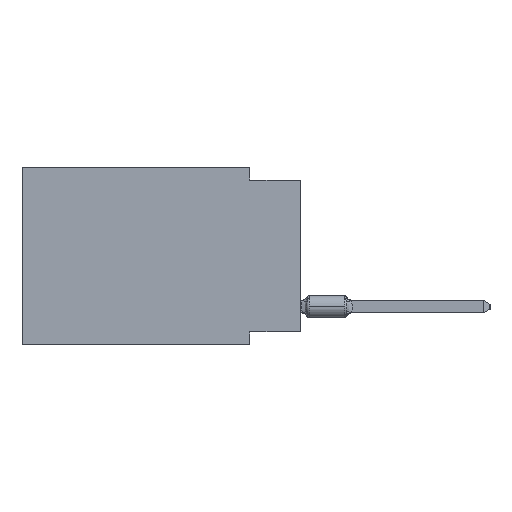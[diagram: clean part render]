
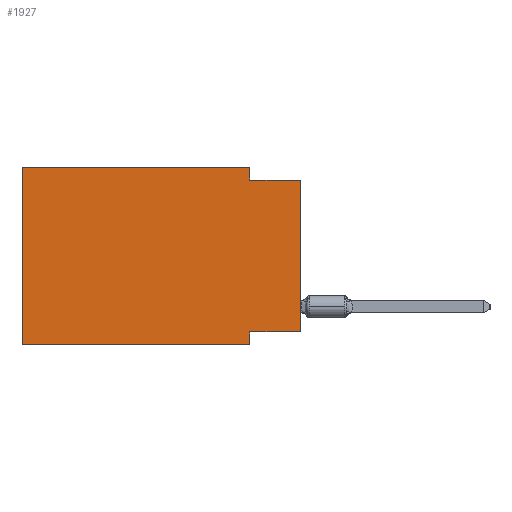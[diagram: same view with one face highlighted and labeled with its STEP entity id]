
A CAD part, left-side view. The second image highlights one B-rep face of the part: STEP entity #1927.
In plain terms, the highlighted planar face has unit normal (-1, 0, 0).
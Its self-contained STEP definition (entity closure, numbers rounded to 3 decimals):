
#405 = CARTESIAN_POINT ( 'NONE',  ( 0., 13.97, 0. ) ) ;
#602 = VECTOR ( 'NONE', #10514, 1000. ) ;
#1927 = ADVANCED_FACE ( 'NONE', ( #8157 ), #25574, .F. ) ;
#2045 = AXIS2_PLACEMENT_3D ( 'NONE', #12859, #8433, #4004 ) ;
#3467 = EDGE_CURVE ( 'NONE', #17275, #5805, #4406, .T. ) ;
#3795 = ORIENTED_EDGE ( 'NONE', *, *, #14991, .F. ) ;
#3963 = DIRECTION ( 'NONE',  ( 0., -1., 0. ) ) ;
#4004 = DIRECTION ( 'NONE',  ( 0., 0., -1. ) ) ;
#4112 = ORIENTED_EDGE ( 'NONE', *, *, #22941, .F. ) ;
#4251 = EDGE_CURVE ( 'NONE', #5805, #24620, #11693, .T. ) ;
#4406 = LINE ( 'NONE', #10503, #20689 ) ;
#4464 = ORIENTED_EDGE ( 'NONE', *, *, #23027, .F. ) ;
#4549 = LINE ( 'NONE', #8986, #602 ) ;
#4824 = CARTESIAN_POINT ( 'NONE',  ( 0., 2.54, -8.89 ) ) ;
#5795 = LINE ( 'NONE', #10486, #11749 ) ;
#5805 = VERTEX_POINT ( 'NONE', #18101 ) ;
#6042 = LINE ( 'NONE', #22933, #11833 ) ;
#6644 = VECTOR ( 'NONE', #8421, 1000. ) ;
#7253 = VECTOR ( 'NONE', #12324, 1000. ) ;
#7646 = ORIENTED_EDGE ( 'NONE', *, *, #23151, .T. ) ;
#7904 = CARTESIAN_POINT ( 'NONE',  ( 0., 2.54, 0. ) ) ;
#8157 = FACE_OUTER_BOUND ( 'NONE', #25905, .T. ) ;
#8173 = LINE ( 'NONE', #7904, #7253 ) ;
#8421 = DIRECTION ( 'NONE',  ( 0., 0., 1. ) ) ;
#8433 = DIRECTION ( 'NONE',  ( 1., 0., 0. ) ) ;
#8986 = CARTESIAN_POINT ( 'NONE',  ( 0., 13.97, -8.89 ) ) ;
#10387 = ORIENTED_EDGE ( 'NONE', *, *, #24903, .T. ) ;
#10486 = CARTESIAN_POINT ( 'NONE',  ( 0., 0., 0. ) ) ;
#10503 = CARTESIAN_POINT ( 'NONE',  ( 0., 0., -8.255 ) ) ;
#10514 = DIRECTION ( 'NONE',  ( 0., -1., 0. ) ) ;
#11693 = LINE ( 'NONE', #15861, #21605 ) ;
#11749 = VECTOR ( 'NONE', #27346, 1000. ) ;
#11811 = ORIENTED_EDGE ( 'NONE', *, *, #4251, .F. ) ;
#11833 = VECTOR ( 'NONE', #3963, 1000. ) ;
#12324 = DIRECTION ( 'NONE',  ( 0., 0., -1. ) ) ;
#12859 = CARTESIAN_POINT ( 'NONE',  ( 0., 13.97, 0. ) ) ;
#12860 = DIRECTION ( 'NONE',  ( 0., 1., 0. ) ) ;
#14485 = CARTESIAN_POINT ( 'NONE',  ( 0., 2.54, -0.635 ) ) ;
#14671 = DIRECTION ( 'NONE',  ( 0., -1., 0. ) ) ;
#14783 = CARTESIAN_POINT ( 'NONE',  ( 0., 13.97, 0. ) ) ;
#14882 = VERTEX_POINT ( 'NONE', #14485 ) ;
#14991 = EDGE_CURVE ( 'NONE', #18155, #26142, #6042, .T. ) ;
#15861 = CARTESIAN_POINT ( 'NONE',  ( 0., 2.54, -8.89 ) ) ;
#16472 = LINE ( 'NONE', #22581, #19612 ) ;
#16500 = CARTESIAN_POINT ( 'NONE',  ( 0., 0., -0.635 ) ) ;
#17275 = VERTEX_POINT ( 'NONE', #23997 ) ;
#18101 = CARTESIAN_POINT ( 'NONE',  ( 0., 2.54, -8.255 ) ) ;
#18155 = VERTEX_POINT ( 'NONE', #405 ) ;
#18309 = ORIENTED_EDGE ( 'NONE', *, *, #19521, .F. ) ;
#18693 = CARTESIAN_POINT ( 'NONE',  ( 0., 2.54, 0. ) ) ;
#18930 = LINE ( 'NONE', #14783, #6644 ) ;
#19521 = EDGE_CURVE ( 'NONE', #24558, #18155, #18930, .T. ) ;
#19612 = VECTOR ( 'NONE', #14671, 1000. ) ;
#20689 = VECTOR ( 'NONE', #12860, 1000. ) ;
#21409 = VERTEX_POINT ( 'NONE', #16500 ) ;
#21605 = VECTOR ( 'NONE', #21944, 1000. ) ;
#21944 = DIRECTION ( 'NONE',  ( 0., 0., -1. ) ) ;
#22581 = CARTESIAN_POINT ( 'NONE',  ( 0., 0., -0.635 ) ) ;
#22933 = CARTESIAN_POINT ( 'NONE',  ( 0., 13.97, 0. ) ) ;
#22941 = EDGE_CURVE ( 'NONE', #26142, #14882, #8173, .T. ) ;
#23027 = EDGE_CURVE ( 'NONE', #14882, #21409, #16472, .T. ) ;
#23151 = EDGE_CURVE ( 'NONE', #24558, #24620, #4549, .T. ) ;
#23467 = ORIENTED_EDGE ( 'NONE', *, *, #3467, .F. ) ;
#23997 = CARTESIAN_POINT ( 'NONE',  ( 0., 0., -8.255 ) ) ;
#24532 = CARTESIAN_POINT ( 'NONE',  ( 0., 13.97, -8.89 ) ) ;
#24558 = VERTEX_POINT ( 'NONE', #24532 ) ;
#24620 = VERTEX_POINT ( 'NONE', #4824 ) ;
#24903 = EDGE_CURVE ( 'NONE', #17275, #21409, #5795, .T. ) ;
#25574 = PLANE ( 'NONE',  #2045 ) ;
#25905 = EDGE_LOOP ( 'NONE', ( #10387, #4464, #4112, #3795, #18309, #7646, #11811, #23467 ) ) ;
#26142 = VERTEX_POINT ( 'NONE', #18693 ) ;
#27346 = DIRECTION ( 'NONE',  ( 0., 0., 1. ) ) ;
